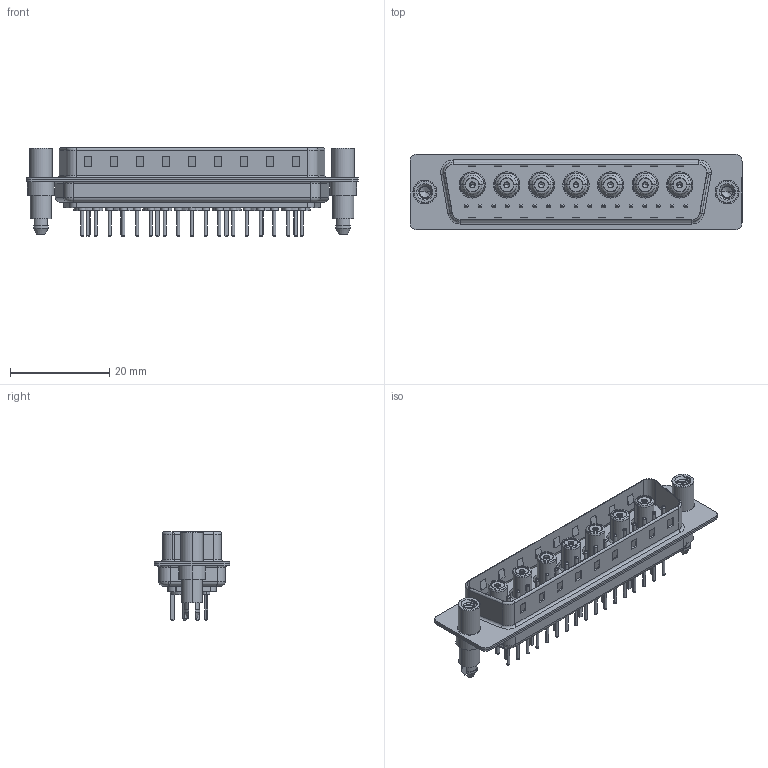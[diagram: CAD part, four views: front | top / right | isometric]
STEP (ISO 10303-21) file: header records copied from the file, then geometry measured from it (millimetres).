
FILE_DESCRIPTION (( 'STEP AP203' ), '1' );
FILE_NAME ('627-24W7624-7T6.STEP', '2019-06-19T01:54:41', ( '' ), ( '' ), 'SwSTEP 2.0', 'SolidWorks 2016', '' );
FILE_SCHEMA (( 'CONFIG_CONTROL_DESIGN' ));
Length unit declared in the file: millimetre
Products named in the file (12): 627-24W7624-7T6; 627Combo Threaded Standoff and Boardlock_6; 627Combo Shell Front_50 Contacts; Co-Ax Jack_Straight PC Tail; Insulator Socket; Insulator Socket 2; Locking Collar; Socket_Str; Co-Ax Jack Assy_St; 627Combo Housing_24W7; 627Combo Contact Row 3_24; 627Combo Shell Rear_50 Contacts
Assembly tree (34 placements, depth 3):
  627-24W7624-7T6
    627Combo Housing_24W7
    627Combo Shell Rear_50 Contacts
    627Combo Shell Front_50 Contacts
    627Combo Threaded Standoff and Boardlock_6  x2
    Co-Ax Jack Assy_St  x7
      Co-Ax Jack_Straight PC Tail
      Insulator Socket
      Insulator Socket 2
      Locking Collar
      Socket_Str
    627Combo Contact Row 3_24  x17
Bounding box: 67 x 15.3 x 17.9 mm (x, y, z)
Volume: 5020.1 mm3; surface area: 13921.6 mm2
Topology: 57 solids, 57 shells, 1870 faces, 4186 edges, 2588 vertices
Faces by surface type: cylinder 736, plane 669, torus 350, cone 81, bspline 20, sphere 14
Entity records: 24125 total; most frequent: CARTESIAN_POINT 4860, DIRECTION 3860, ORIENTED_EDGE 3430, EDGE_CURVE 1715, AXIS2_PLACEMENT_3D 1477, VERTEX_POINT 1095, LINE 906, VECTOR 906
